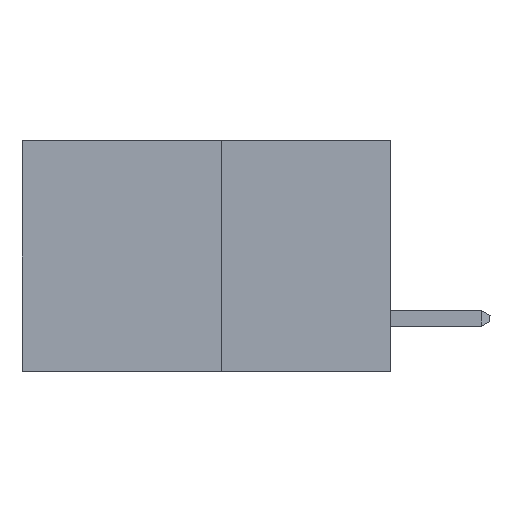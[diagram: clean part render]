
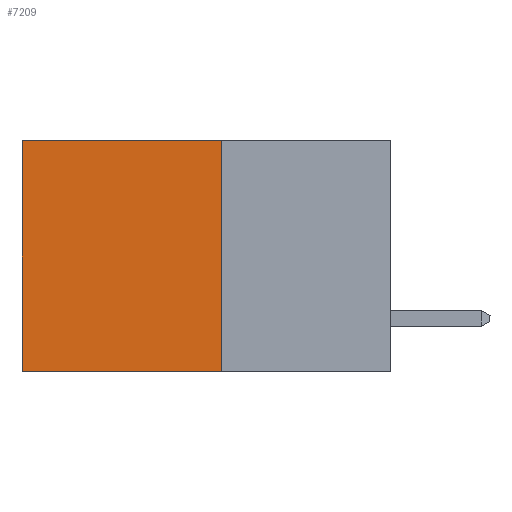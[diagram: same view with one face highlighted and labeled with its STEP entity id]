
A CAD part, left-side view. The second image highlights one B-rep face of the part: STEP entity #7209.
In plain terms, the highlighted planar face has unit normal (-1, 0, 0).
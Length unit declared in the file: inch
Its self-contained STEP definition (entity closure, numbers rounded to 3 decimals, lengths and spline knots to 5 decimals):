
#794 = VECTOR ( 'NONE', #4390, 39.37008 ) ;
#1220 = VECTOR ( 'NONE', #9848, 39.37008 ) ;
#1277 = ORIENTED_EDGE ( 'NONE', *, *, #2285, .T. ) ;
#1289 = AXIS2_PLACEMENT_3D ( 'NONE', #4226, #9762, #5005 ) ;
#1368 = VERTEX_POINT ( 'NONE', #2987 ) ;
#1771 = CARTESIAN_POINT ( 'NONE',  ( 0.277, 0.27, -0.37 ) ) ;
#1809 = VERTEX_POINT ( 'NONE', #7107 ) ;
#1894 = DIRECTION ( 'NONE',  ( 0., 1., 0. ) ) ;
#1971 = CARTESIAN_POINT ( 'NONE',  ( 0.277, 0.27, -0.37 ) ) ;
#2278 = CARTESIAN_POINT ( 'NONE',  ( 0.277, 0.27, 0. ) ) ;
#2285 = EDGE_CURVE ( 'NONE', #1368, #2398, #6927, .T. ) ;
#2398 = VERTEX_POINT ( 'NONE', #6484 ) ;
#2463 = VECTOR ( 'NONE', #1894, 39.37008 ) ;
#2506 = CARTESIAN_POINT ( 'NONE',  ( 0.277, 0.27, -0.37 ) ) ;
#2598 = DIRECTION ( 'NONE',  ( 0., 1., 0. ) ) ;
#2987 = CARTESIAN_POINT ( 'NONE',  ( 0.277, 0.27, 0. ) ) ;
#3276 = ORIENTED_EDGE ( 'NONE', *, *, #5819, .F. ) ;
#3486 = LINE ( 'NONE', #1771, #1220 ) ;
#4226 = CARTESIAN_POINT ( 'NONE',  ( 0.277, 0.27, -0.37 ) ) ;
#4390 = DIRECTION ( 'NONE',  ( 0., 0., -1. ) ) ;
#4891 = VECTOR ( 'NONE', #2598, 39.37008 ) ;
#5005 = DIRECTION ( 'NONE',  ( 0., 0., -1. ) ) ;
#5796 = EDGE_LOOP ( 'NONE', ( #7450, #3276, #7714, #1277 ) ) ;
#5819 = EDGE_CURVE ( 'NONE', #6278, #1809, #8735, .T. ) ;
#6148 = EDGE_CURVE ( 'NONE', #1368, #6278, #3486, .T. ) ;
#6278 = VERTEX_POINT ( 'NONE', #1971 ) ;
#6484 = CARTESIAN_POINT ( 'NONE',  ( 0.277, 0.59, 0. ) ) ;
#6682 = LINE ( 'NONE', #9210, #794 ) ;
#6927 = LINE ( 'NONE', #2278, #2463 ) ;
#7107 = CARTESIAN_POINT ( 'NONE',  ( 0.277, 0.59, -0.37 ) ) ;
#7209 = ADVANCED_FACE ( 'NONE', ( #8009 ), #9041, .F. ) ;
#7297 = EDGE_CURVE ( 'NONE', #2398, #1809, #6682, .T. ) ;
#7450 = ORIENTED_EDGE ( 'NONE', *, *, #7297, .T. ) ;
#7714 = ORIENTED_EDGE ( 'NONE', *, *, #6148, .F. ) ;
#8009 = FACE_OUTER_BOUND ( 'NONE', #5796, .T. ) ;
#8735 = LINE ( 'NONE', #2506, #4891 ) ;
#9041 = PLANE ( 'NONE',  #1289 ) ;
#9210 = CARTESIAN_POINT ( 'NONE',  ( 0.277, 0.59, -0.37 ) ) ;
#9762 = DIRECTION ( 'NONE',  ( 1., 0., 0. ) ) ;
#9848 = DIRECTION ( 'NONE',  ( 0., 0., -1. ) ) ;
